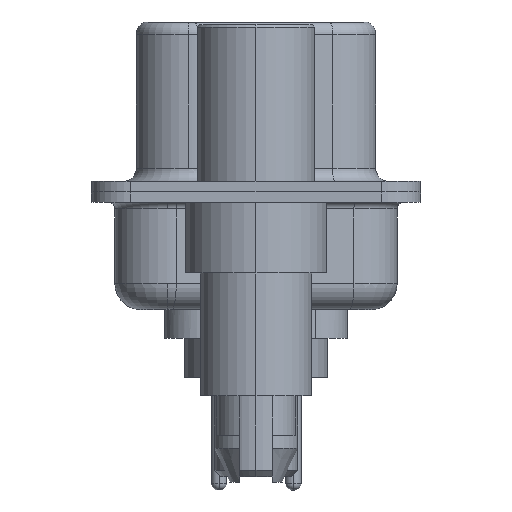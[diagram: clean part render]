
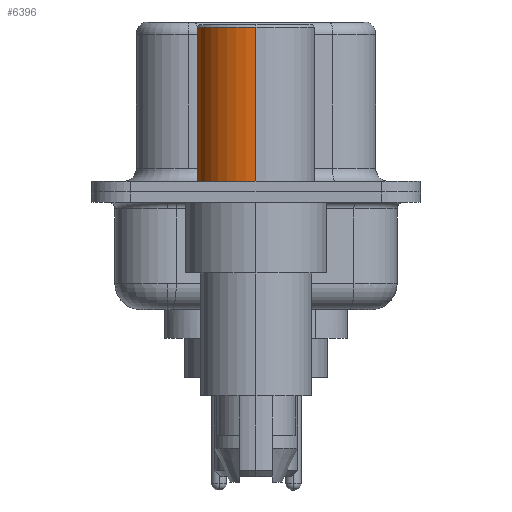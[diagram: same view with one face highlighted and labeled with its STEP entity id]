
A CAD part, left-side view. The second image highlights one B-rep face of the part: STEP entity #6396.
In plain terms, the highlighted cylindrical face has radius 2.25 mm (diameter 4.5 mm), a partial arc.
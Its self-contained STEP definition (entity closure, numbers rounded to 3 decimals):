
#1866 = DIRECTION ( 'NONE',  ( 1., 0., 0. ) ) ;
#2297 = AXIS2_PLACEMENT_3D ( 'NONE', #13413, #9060, #1866 ) ;
#2674 = ORIENTED_EDGE ( 'NONE', *, *, #13467, .F. ) ;
#2785 = ORIENTED_EDGE ( 'NONE', *, *, #6417, .T. ) ;
#3036 = ORIENTED_EDGE ( 'NONE', *, *, #15605, .T. ) ;
#3462 = VERTEX_POINT ( 'NONE', #13232 ) ;
#3484 = VERTEX_POINT ( 'NONE', #7614 ) ;
#6128 = CARTESIAN_POINT ( 'NONE',  ( -2.25, 0., 0.4 ) ) ;
#6396 = ADVANCED_FACE ( 'NONE', ( #14491 ), #17884, .T. ) ;
#6417 = EDGE_CURVE ( 'NONE', #11603, #3484, #6814, .T. ) ;
#6759 = CARTESIAN_POINT ( 'NONE',  ( 0., 0., 0.4 ) ) ;
#6814 = LINE ( 'NONE', #9114, #7275 ) ;
#7028 = DIRECTION ( 'NONE',  ( 0., 0., 1. ) ) ;
#7275 = VECTOR ( 'NONE', #17761, 1000. ) ;
#7614 = CARTESIAN_POINT ( 'NONE',  ( -2.25, 0., 6.3 ) ) ;
#8210 = DIRECTION ( 'NONE',  ( 1., 0., 0. ) ) ;
#8973 = VERTEX_POINT ( 'NONE', #16916 ) ;
#9060 = DIRECTION ( 'NONE',  ( 0., 0., 1. ) ) ;
#9114 = CARTESIAN_POINT ( 'NONE',  ( -2.25, 0., 0.581 ) ) ;
#9632 = DIRECTION ( 'NONE',  ( 0., 0., 1. ) ) ;
#10763 = AXIS2_PLACEMENT_3D ( 'NONE', #6759, #16853, #8210 ) ;
#11362 = EDGE_CURVE ( 'NONE', #3462, #3484, #15715, .T. ) ;
#11509 = VECTOR ( 'NONE', #9632, 1000. ) ;
#11603 = VERTEX_POINT ( 'NONE', #6128 ) ;
#13232 = CARTESIAN_POINT ( 'NONE',  ( 2.25, 0., 6.3 ) ) ;
#13413 = CARTESIAN_POINT ( 'NONE',  ( 0., 0., 0.581 ) ) ;
#13467 = EDGE_CURVE ( 'NONE', #8973, #3462, #15324, .T. ) ;
#14491 = FACE_OUTER_BOUND ( 'NONE', #16608, .T. ) ;
#15268 = CIRCLE ( 'NONE', #10763, 2.25 ) ;
#15324 = LINE ( 'NONE', #16805, #11509 ) ;
#15605 = EDGE_CURVE ( 'NONE', #8973, #11603, #15268, .T. ) ;
#15664 = CARTESIAN_POINT ( 'NONE',  ( 0., 0., 6.3 ) ) ;
#15715 = CIRCLE ( 'NONE', #18683, 2.25 ) ;
#16608 = EDGE_LOOP ( 'NONE', ( #3036, #2785, #18039, #2674 ) ) ;
#16805 = CARTESIAN_POINT ( 'NONE',  ( 2.25, 0., 0.581 ) ) ;
#16853 = DIRECTION ( 'NONE',  ( 0., 0., 1. ) ) ;
#16916 = CARTESIAN_POINT ( 'NONE',  ( 2.25, 0., 0.4 ) ) ;
#17109 = DIRECTION ( 'NONE',  ( 1., 0., 0. ) ) ;
#17761 = DIRECTION ( 'NONE',  ( 0., 0., 1. ) ) ;
#17884 = CYLINDRICAL_SURFACE ( 'NONE', #2297, 2.25 ) ;
#18039 = ORIENTED_EDGE ( 'NONE', *, *, #11362, .F. ) ;
#18683 = AXIS2_PLACEMENT_3D ( 'NONE', #15664, #7028, #17109 ) ;
